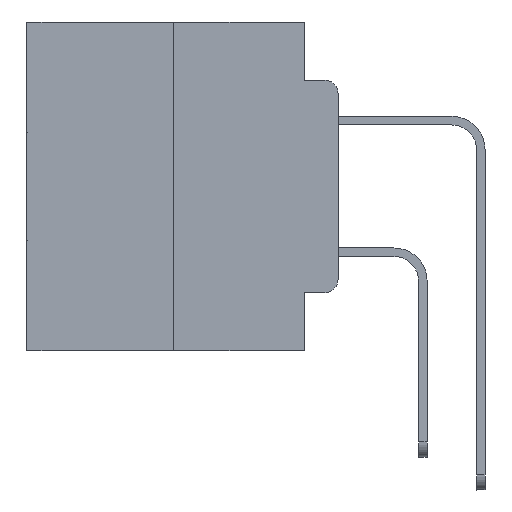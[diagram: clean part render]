
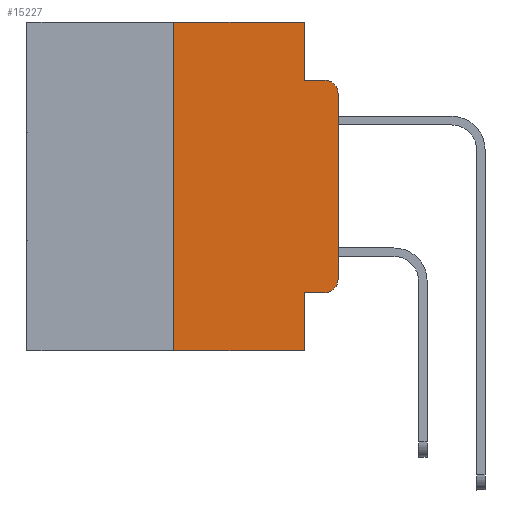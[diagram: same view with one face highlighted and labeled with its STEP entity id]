
A CAD part, left-side view. The second image highlights one B-rep face of the part: STEP entity #15227.
In plain terms, the highlighted planar face has unit normal (-1, 0, 0).
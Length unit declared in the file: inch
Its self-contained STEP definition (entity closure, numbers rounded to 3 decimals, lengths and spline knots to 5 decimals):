
#95 = EDGE_CURVE ( 'NONE', #23463, #24855, #2704, .T. ) ;
#683 = AXIS2_PLACEMENT_3D ( 'NONE', #6396, #1788, #9285 ) ;
#1095 = DIRECTION ( 'NONE',  ( 0., -1., 0. ) ) ;
#1788 = DIRECTION ( 'NONE',  ( -1., 0., 0. ) ) ;
#2001 = VECTOR ( 'NONE', #29071, 39.37008 ) ;
#2080 = CARTESIAN_POINT ( 'NONE',  ( 0., 0., -0.1085 ) ) ;
#2135 = EDGE_CURVE ( 'NONE', #20213, #19793, #21791, .T. ) ;
#2704 = LINE ( 'NONE', #25220, #2001 ) ;
#3208 = VECTOR ( 'NONE', #19164, 39.37008 ) ;
#3525 = DIRECTION ( 'NONE',  ( 0., 0., 1. ) ) ;
#4018 = ORIENTED_EDGE ( 'NONE', *, *, #95, .F. ) ;
#4677 = LINE ( 'NONE', #7931, #3208 ) ;
#5099 = ORIENTED_EDGE ( 'NONE', *, *, #27545, .T. ) ;
#5705 = LINE ( 'NONE', #28183, #10335 ) ;
#5708 = DIRECTION ( 'NONE',  ( 1., 0., 0. ) ) ;
#6105 = VECTOR ( 'NONE', #9520, 39.37008 ) ;
#6396 = CARTESIAN_POINT ( 'NONE',  ( 0., 0.02, -0.1085 ) ) ;
#6804 = LINE ( 'NONE', #7207, #6105 ) ;
#6812 = EDGE_CURVE ( 'NONE', #27144, #28478, #28480, .T. ) ;
#6871 = EDGE_CURVE ( 'NONE', #10596, #25455, #21201, .T. ) ;
#7207 = CARTESIAN_POINT ( 'NONE',  ( 0., 0.051, -0.0885 ) ) ;
#7561 = ORIENTED_EDGE ( 'NONE', *, *, #2135, .T. ) ;
#7577 = CARTESIAN_POINT ( 'NONE',  ( 0., 0.051, -0.4115 ) ) ;
#7704 = CARTESIAN_POINT ( 'NONE',  ( 0., 0.25, 0. ) ) ;
#7931 = CARTESIAN_POINT ( 'NONE',  ( 0., 0., 0. ) ) ;
#8852 = VERTEX_POINT ( 'NONE', #9007 ) ;
#9007 = CARTESIAN_POINT ( 'NONE',  ( 0., 0.051, -0.0885 ) ) ;
#9285 = DIRECTION ( 'NONE',  ( 0., 0., -1. ) ) ;
#9520 = DIRECTION ( 'NONE',  ( 0., -1., 0. ) ) ;
#9691 = FACE_OUTER_BOUND ( 'NONE', #17688, .T. ) ;
#10049 = ORIENTED_EDGE ( 'NONE', *, *, #11438, .F. ) ;
#10234 = DIRECTION ( 'NONE',  ( 0., -1., 0. ) ) ;
#10335 = VECTOR ( 'NONE', #26178, 39.37008 ) ;
#10596 = VERTEX_POINT ( 'NONE', #13219 ) ;
#11048 = EDGE_CURVE ( 'NONE', #28478, #18390, #27926, .T. ) ;
#11065 = EDGE_CURVE ( 'NONE', #27144, #24855, #27258, .T. ) ;
#11070 = EDGE_CURVE ( 'NONE', #25455, #20213, #4677, .T. ) ;
#11223 = ORIENTED_EDGE ( 'NONE', *, *, #6871, .T. ) ;
#11438 = EDGE_CURVE ( 'NONE', #8852, #19793, #6804, .T. ) ;
#11600 = VECTOR ( 'NONE', #25630, 39.37008 ) ;
#11918 = CARTESIAN_POINT ( 'NONE',  ( 0., 0.051, -0.4115 ) ) ;
#12491 = CARTESIAN_POINT ( 'NONE',  ( 0., 0.051, 0. ) ) ;
#12797 = AXIS2_PLACEMENT_3D ( 'NONE', #12950, #28560, #15280 ) ;
#12950 = CARTESIAN_POINT ( 'NONE',  ( 0., 0.02, -0.3915 ) ) ;
#13219 = CARTESIAN_POINT ( 'NONE',  ( 0., 0.02, -0.4115 ) ) ;
#14765 = ORIENTED_EDGE ( 'NONE', *, *, #24972, .F. ) ;
#14836 = CARTESIAN_POINT ( 'NONE',  ( 0., 0.473, 0. ) ) ;
#15227 = ADVANCED_FACE ( 'NONE', ( #9691 ), #19307, .F. ) ;
#15280 = DIRECTION ( 'NONE',  ( 0., 0., -1. ) ) ;
#15452 = VECTOR ( 'NONE', #1095, 39.37008 ) ;
#15509 = ORIENTED_EDGE ( 'NONE', *, *, #6812, .F. ) ;
#16141 = VECTOR ( 'NONE', #10234, 39.37008 ) ;
#17257 = ORIENTED_EDGE ( 'NONE', *, *, #11065, .T. ) ;
#17679 = LINE ( 'NONE', #7577, #11600 ) ;
#17688 = EDGE_LOOP ( 'NONE', ( #18627, #7561, #10049, #14765, #27988, #15509, #17257, #4018, #5099, #11223 ) ) ;
#18390 = VERTEX_POINT ( 'NONE', #12491 ) ;
#18627 = ORIENTED_EDGE ( 'NONE', *, *, #11070, .T. ) ;
#19164 = DIRECTION ( 'NONE',  ( 0., 0., 1. ) ) ;
#19307 = PLANE ( 'NONE',  #25140 ) ;
#19793 = VERTEX_POINT ( 'NONE', #25567 ) ;
#20213 = VERTEX_POINT ( 'NONE', #2080 ) ;
#21201 = CIRCLE ( 'NONE', #12797, 0.02 ) ;
#21497 = CARTESIAN_POINT ( 'NONE',  ( 0., 0.473, 0. ) ) ;
#21546 = DIRECTION ( 'NONE',  ( 0., 0., -1. ) ) ;
#21676 = CARTESIAN_POINT ( 'NONE',  ( 0., 0., -0.3915 ) ) ;
#21791 = CIRCLE ( 'NONE', #683, 0.02 ) ;
#21959 = CARTESIAN_POINT ( 'NONE',  ( 0., 0.25, -0.5 ) ) ;
#23280 = VECTOR ( 'NONE', #3525, 39.37008 ) ;
#23463 = VERTEX_POINT ( 'NONE', #11918 ) ;
#23910 = CARTESIAN_POINT ( 'NONE',  ( 0., 0.25, 0. ) ) ;
#24855 = VERTEX_POINT ( 'NONE', #27977 ) ;
#24972 = EDGE_CURVE ( 'NONE', #18390, #8852, #5705, .T. ) ;
#25140 = AXIS2_PLACEMENT_3D ( 'NONE', #14836, #5708, #21546 ) ;
#25220 = CARTESIAN_POINT ( 'NONE',  ( 0., 0.051, 0. ) ) ;
#25455 = VERTEX_POINT ( 'NONE', #21676 ) ;
#25567 = CARTESIAN_POINT ( 'NONE',  ( 0., 0.02, -0.0885 ) ) ;
#25630 = DIRECTION ( 'NONE',  ( 0., -1., 0. ) ) ;
#26178 = DIRECTION ( 'NONE',  ( 0., 0., -1. ) ) ;
#27144 = VERTEX_POINT ( 'NONE', #21959 ) ;
#27258 = LINE ( 'NONE', #28174, #15452 ) ;
#27545 = EDGE_CURVE ( 'NONE', #23463, #10596, #17679, .T. ) ;
#27926 = LINE ( 'NONE', #21497, #16141 ) ;
#27977 = CARTESIAN_POINT ( 'NONE',  ( 0., 0.051, -0.5 ) ) ;
#27988 = ORIENTED_EDGE ( 'NONE', *, *, #11048, .F. ) ;
#28174 = CARTESIAN_POINT ( 'NONE',  ( 0., 0.473, -0.5 ) ) ;
#28183 = CARTESIAN_POINT ( 'NONE',  ( 0., 0.051, 0. ) ) ;
#28478 = VERTEX_POINT ( 'NONE', #7704 ) ;
#28480 = LINE ( 'NONE', #23910, #23280 ) ;
#28560 = DIRECTION ( 'NONE',  ( -1., 0., 0. ) ) ;
#29071 = DIRECTION ( 'NONE',  ( 0., 0., -1. ) ) ;
